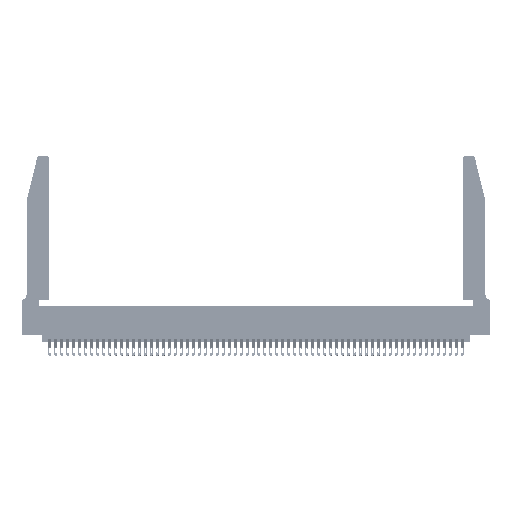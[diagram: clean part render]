
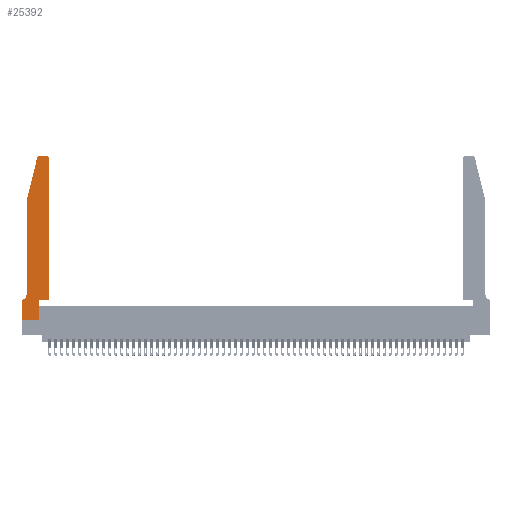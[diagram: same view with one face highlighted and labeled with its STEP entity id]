
A CAD part, top view. The second image highlights one B-rep face of the part: STEP entity #25392.
In plain terms, the highlighted planar face has unit normal (0, 0, 1).
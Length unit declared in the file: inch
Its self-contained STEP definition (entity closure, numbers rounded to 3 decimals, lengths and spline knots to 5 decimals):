
#77 = VECTOR ( 'NONE', #45039, 39.37008 ) ;
#799 = DIRECTION ( 'NONE',  ( 0., 0., 1. ) ) ;
#1338 = CARTESIAN_POINT ( 'NONE',  ( 0., 0., 0.37 ) ) ;
#1482 = VERTEX_POINT ( 'NONE', #1550 ) ;
#1550 = CARTESIAN_POINT ( 'NONE',  ( 0.25487, 2.72718, 0.37 ) ) ;
#2487 = VERTEX_POINT ( 'NONE', #5713 ) ;
#3979 = CARTESIAN_POINT ( 'NONE',  ( 0.0055, 0.42, 0.37 ) ) ;
#5148 = VERTEX_POINT ( 'NONE', #20136 ) ;
#5175 = DIRECTION ( 'NONE',  ( 1., 0., 0. ) ) ;
#5474 = LINE ( 'NONE', #7550, #8188 ) ;
#5628 = AXIS2_PLACEMENT_3D ( 'NONE', #27060, #18671, #49513 ) ;
#5713 = CARTESIAN_POINT ( 'NONE',  ( 0.2865, 0., 0.37 ) ) ;
#6047 = CARTESIAN_POINT ( 'NONE',  ( 0.284, 2.75, 0.37 ) ) ;
#6105 = EDGE_CURVE ( 'NONE', #1482, #27310, #38319, .T. ) ;
#6182 = VECTOR ( 'NONE', #8650, 39.37008 ) ;
#6184 = CARTESIAN_POINT ( 'NONE',  ( 0.0755, 2., 0.37 ) ) ;
#6729 = VERTEX_POINT ( 'NONE', #6047 ) ;
#7550 = CARTESIAN_POINT ( 'NONE',  ( 0.0755, 2., 0.37 ) ) ;
#8188 = VECTOR ( 'NONE', #46403, 39.37008 ) ;
#8501 = DIRECTION ( 'NONE',  ( 0., 0., -1. ) ) ;
#8650 = DIRECTION ( 'NONE',  ( 1., 0., 0. ) ) ;
#10412 = VECTOR ( 'NONE', #36383, 39.37008 ) ;
#10642 = CARTESIAN_POINT ( 'NONE',  ( 0.0755, 0.42, 0.37 ) ) ;
#11700 = EDGE_CURVE ( 'NONE', #27310, #52637, #5474, .T. ) ;
#11864 = DIRECTION ( 'NONE',  ( 0., 1., 0. ) ) ;
#12579 = EDGE_CURVE ( 'NONE', #2487, #30834, #44167, .T. ) ;
#12776 = VECTOR ( 'NONE', #42004, 39.37008 ) ;
#12819 = ORIENTED_EDGE ( 'NONE', *, *, #30049, .T. ) ;
#14163 = VERTEX_POINT ( 'NONE', #31640 ) ;
#15188 = AXIS2_PLACEMENT_3D ( 'NONE', #48948, #49324, #18488 ) ;
#17518 = EDGE_CURVE ( 'NONE', #30834, #41824, #18424, .T. ) ;
#18424 = LINE ( 'NONE', #38730, #6182 ) ;
#18488 = DIRECTION ( 'NONE',  ( 1., 0., 0. ) ) ;
#18671 = DIRECTION ( 'NONE',  ( 0., 0., 1. ) ) ;
#18761 = CARTESIAN_POINT ( 'NONE',  ( 0., 0., 0.37 ) ) ;
#19529 = CARTESIAN_POINT ( 'NONE',  ( 0.0755, 0.35, 0.37 ) ) ;
#20136 = CARTESIAN_POINT ( 'NONE',  ( 0.0055, 0.35, 0.37 ) ) ;
#20316 = LINE ( 'NONE', #55881, #23699 ) ;
#20425 = VERTEX_POINT ( 'NONE', #35650 ) ;
#20572 = LINE ( 'NONE', #18761, #77 ) ;
#20903 = EDGE_LOOP ( 'NONE', ( #12819, #24767, #38625, #26597, #40270, #25891, #41538, #43000, #41687, #26468, #44243, #55961 ) ) ;
#21159 = VECTOR ( 'NONE', #22840, 39.37008 ) ;
#21344 = FACE_OUTER_BOUND ( 'NONE', #20903, .T. ) ;
#22483 = PLANE ( 'NONE',  #29926 ) ;
#22840 = DIRECTION ( 'NONE',  ( 1., 0., 0. ) ) ;
#23035 = VECTOR ( 'NONE', #30650, 39.37008 ) ;
#23699 = VECTOR ( 'NONE', #11864, 39.37008 ) ;
#24767 = ORIENTED_EDGE ( 'NONE', *, *, #52455, .T. ) ;
#25392 = ADVANCED_FACE ( 'NONE', ( #21344 ), #22483, .T. ) ;
#25891 = ORIENTED_EDGE ( 'NONE', *, *, #29752, .T. ) ;
#26173 = CARTESIAN_POINT ( 'NONE',  ( 0.0755, 2., 0.37 ) ) ;
#26468 = ORIENTED_EDGE ( 'NONE', *, *, #17518, .T. ) ;
#26597 = ORIENTED_EDGE ( 'NONE', *, *, #11700, .T. ) ;
#26707 = AXIS2_PLACEMENT_3D ( 'NONE', #3979, #8501, #38962 ) ;
#26764 = VERTEX_POINT ( 'NONE', #27222 ) ;
#26866 = CARTESIAN_POINT ( 'NONE',  ( 0., 0.35, 0.37 ) ) ;
#27003 = EDGE_CURVE ( 'NONE', #52637, #5148, #41639, .T. ) ;
#27060 = CARTESIAN_POINT ( 'NONE',  ( 0.284, 2.72, 0.37 ) ) ;
#27195 = EDGE_CURVE ( 'NONE', #45189, #14163, #20572, .T. ) ;
#27222 = CARTESIAN_POINT ( 'NONE',  ( 0.4205, 2.75, 0.37 ) ) ;
#27310 = VERTEX_POINT ( 'NONE', #6184 ) ;
#29666 = CARTESIAN_POINT ( 'NONE',  ( 0.4505, 0.35, 0.37 ) ) ;
#29752 = EDGE_CURVE ( 'NONE', #5148, #45189, #48917, .T. ) ;
#29926 = AXIS2_PLACEMENT_3D ( 'NONE', #26866, #799, #5175 ) ;
#29976 = LINE ( 'NONE', #1338, #21159 ) ;
#30049 = EDGE_CURVE ( 'NONE', #26764, #6729, #55718, .T. ) ;
#30377 = CIRCLE ( 'NONE', #15188, 0.03 ) ;
#30650 = DIRECTION ( 'NONE',  ( 0., 1., 0. ) ) ;
#30720 = EDGE_CURVE ( 'NONE', #20425, #26764, #30377, .T. ) ;
#30834 = VERTEX_POINT ( 'NONE', #49889 ) ;
#31299 = CARTESIAN_POINT ( 'NONE',  ( 0.2605, 2.75, 0.37 ) ) ;
#31640 = CARTESIAN_POINT ( 'NONE',  ( 0., 0., 0.37 ) ) ;
#33341 = CARTESIAN_POINT ( 'NONE',  ( 0., 0.35, 0.37 ) ) ;
#34084 = EDGE_CURVE ( 'NONE', #14163, #2487, #29976, .T. ) ;
#35650 = CARTESIAN_POINT ( 'NONE',  ( 0.4505, 2.72, 0.37 ) ) ;
#36383 = DIRECTION ( 'NONE',  ( -0.239, -0.971, 0. ) ) ;
#38319 = LINE ( 'NONE', #26173, #10412 ) ;
#38625 = ORIENTED_EDGE ( 'NONE', *, *, #6105, .T. ) ;
#38730 = CARTESIAN_POINT ( 'NONE',  ( 0.4505, 0.35, 0.37 ) ) ;
#38962 = DIRECTION ( 'NONE',  ( -1., 0., 0. ) ) ;
#40270 = ORIENTED_EDGE ( 'NONE', *, *, #27003, .T. ) ;
#41372 = VECTOR ( 'NONE', #52044, 39.37008 ) ;
#41538 = ORIENTED_EDGE ( 'NONE', *, *, #27195, .T. ) ;
#41639 = CIRCLE ( 'NONE', #26707, 0.07 ) ;
#41687 = ORIENTED_EDGE ( 'NONE', *, *, #12579, .T. ) ;
#41824 = VERTEX_POINT ( 'NONE', #29666 ) ;
#42004 = DIRECTION ( 'NONE',  ( -1., 0., 0. ) ) ;
#43000 = ORIENTED_EDGE ( 'NONE', *, *, #34084, .T. ) ;
#44167 = LINE ( 'NONE', #52172, #23035 ) ;
#44243 = ORIENTED_EDGE ( 'NONE', *, *, #46680, .T. ) ;
#45039 = DIRECTION ( 'NONE',  ( 0., -1., 0. ) ) ;
#45189 = VERTEX_POINT ( 'NONE', #33341 ) ;
#46403 = DIRECTION ( 'NONE',  ( 0., -1., 0. ) ) ;
#46680 = EDGE_CURVE ( 'NONE', #41824, #20425, #20316, .T. ) ;
#48917 = LINE ( 'NONE', #19529, #12776 ) ;
#48948 = CARTESIAN_POINT ( 'NONE',  ( 0.4205, 2.72, 0.37 ) ) ;
#49324 = DIRECTION ( 'NONE',  ( 0., 0., 1. ) ) ;
#49383 = CIRCLE ( 'NONE', #5628, 0.03 ) ;
#49513 = DIRECTION ( 'NONE',  ( 1., 0., 0. ) ) ;
#49889 = CARTESIAN_POINT ( 'NONE',  ( 0.2865, 0.35, 0.37 ) ) ;
#52044 = DIRECTION ( 'NONE',  ( -1., 0., 0. ) ) ;
#52172 = CARTESIAN_POINT ( 'NONE',  ( 0.2865, 0.35, 0.37 ) ) ;
#52455 = EDGE_CURVE ( 'NONE', #6729, #1482, #49383, .T. ) ;
#52637 = VERTEX_POINT ( 'NONE', #10642 ) ;
#55718 = LINE ( 'NONE', #31299, #41372 ) ;
#55881 = CARTESIAN_POINT ( 'NONE',  ( 0.4505, 0.35, 0.37 ) ) ;
#55961 = ORIENTED_EDGE ( 'NONE', *, *, #30720, .T. ) ;
